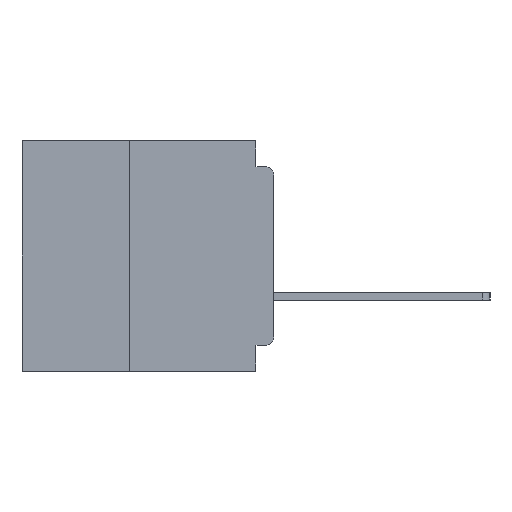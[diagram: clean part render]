
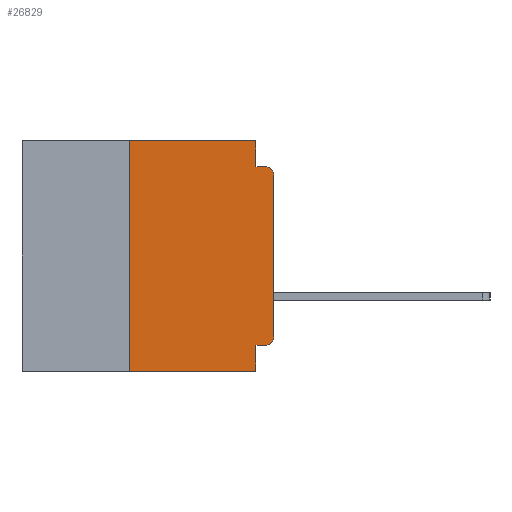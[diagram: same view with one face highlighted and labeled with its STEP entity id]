
A CAD part, left-side view. The second image highlights one B-rep face of the part: STEP entity #26829.
In plain terms, the highlighted planar face has unit normal (-1, 0, 0).
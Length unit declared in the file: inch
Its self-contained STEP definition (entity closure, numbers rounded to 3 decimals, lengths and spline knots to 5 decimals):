
#3 = VERTEX_POINT ( 'NONE', #35363 ) ;
#41 = EDGE_CURVE ( 'NONE', #34626, #41561, #30622, .T. ) ;
#178 = ORIENTED_EDGE ( 'NONE', *, *, #27893, .F. ) ;
#1180 = CARTESIAN_POINT ( 'NONE',  ( 0., 0., -0.06 ) ) ;
#1200 = DIRECTION ( 'NONE',  ( 0., 0., -1. ) ) ;
#1345 = VERTEX_POINT ( 'NONE', #44068 ) ;
#2006 = ORIENTED_EDGE ( 'NONE', *, *, #9228, .F. ) ;
#2143 = CARTESIAN_POINT ( 'NONE',  ( 0., 0.031, 0. ) ) ;
#2938 = EDGE_LOOP ( 'NONE', ( #5595, #6487, #9925, #178, #2006, #3854, #11358, #15460, #45734, #35679 ) ) ;
#3104 = DIRECTION ( 'NONE',  ( 0., 1., 0. ) ) ;
#3542 = VECTOR ( 'NONE', #44884, 39.37008 ) ;
#3665 = DIRECTION ( 'NONE',  ( 1., 0., 0. ) ) ;
#3854 = ORIENTED_EDGE ( 'NONE', *, *, #25334, .F. ) ;
#4952 = VERTEX_POINT ( 'NONE', #33995 ) ;
#5595 = ORIENTED_EDGE ( 'NONE', *, *, #14968, .T. ) ;
#6020 = LINE ( 'NONE', #2143, #12818 ) ;
#6022 = LINE ( 'NONE', #37844, #16567 ) ;
#6487 = ORIENTED_EDGE ( 'NONE', *, *, #41, .T. ) ;
#7938 = VERTEX_POINT ( 'NONE', #29841 ) ;
#8248 = CARTESIAN_POINT ( 'NONE',  ( 0., 0.015, -0.06 ) ) ;
#9228 = EDGE_CURVE ( 'NONE', #7938, #15214, #11077, .T. ) ;
#9925 = ORIENTED_EDGE ( 'NONE', *, *, #34168, .F. ) ;
#10489 = CARTESIAN_POINT ( 'NONE',  ( 0., 0., 0. ) ) ;
#10642 = EDGE_CURVE ( 'NONE', #3, #43529, #35907, .T. ) ;
#11077 = LINE ( 'NONE', #41957, #29340 ) ;
#11358 = ORIENTED_EDGE ( 'NONE', *, *, #14880, .T. ) ;
#12048 = CARTESIAN_POINT ( 'NONE',  ( 0., 0.031, 0. ) ) ;
#12239 = EDGE_CURVE ( 'NONE', #43529, #1345, #24735, .T. ) ;
#12464 = DIRECTION ( 'NONE',  ( -1., 0., 0. ) ) ;
#12818 = VECTOR ( 'NONE', #44821, 39.37008 ) ;
#13395 = CARTESIAN_POINT ( 'NONE',  ( 0., 0., -0.34 ) ) ;
#14012 = VECTOR ( 'NONE', #3104, 39.37008 ) ;
#14355 = LINE ( 'NONE', #20698, #33811 ) ;
#14684 = CARTESIAN_POINT ( 'NONE',  ( 0., 0., -0.355 ) ) ;
#14880 = EDGE_CURVE ( 'NONE', #29068, #1345, #24453, .T. ) ;
#14968 = EDGE_CURVE ( 'NONE', #15480, #34626, #40204, .T. ) ;
#15214 = VERTEX_POINT ( 'NONE', #12048 ) ;
#15460 = ORIENTED_EDGE ( 'NONE', *, *, #12239, .F. ) ;
#15480 = VERTEX_POINT ( 'NONE', #13395 ) ;
#15895 = CARTESIAN_POINT ( 'NONE',  ( 0., 0.015, -0.34 ) ) ;
#16567 = VECTOR ( 'NONE', #41550, 39.37008 ) ;
#17595 = CARTESIAN_POINT ( 'NONE',  ( 0., 0.25, -0.4 ) ) ;
#19838 = DIRECTION ( 'NONE',  ( 0., 0., -1. ) ) ;
#20698 = CARTESIAN_POINT ( 'NONE',  ( 0., 0.25, -0.4 ) ) ;
#20819 = VECTOR ( 'NONE', #33852, 39.37008 ) ;
#22520 = AXIS2_PLACEMENT_3D ( 'NONE', #8248, #12464, #36124 ) ;
#23288 = PLANE ( 'NONE',  #43903 ) ;
#23530 = VECTOR ( 'NONE', #1200, 39.37008 ) ;
#23968 = FACE_OUTER_BOUND ( 'NONE', #2938, .T. ) ;
#24453 = LINE ( 'NONE', #29423, #3542 ) ;
#24594 = DIRECTION ( 'NONE',  ( 0., 0., 1. ) ) ;
#24735 = LINE ( 'NONE', #36448, #23530 ) ;
#25334 = EDGE_CURVE ( 'NONE', #29068, #7938, #14355, .T. ) ;
#26829 = ADVANCED_FACE ( 'NONE', ( #23968 ), #23288, .F. ) ;
#27163 = CARTESIAN_POINT ( 'NONE',  ( 0., 0.437, 0. ) ) ;
#27893 = EDGE_CURVE ( 'NONE', #15214, #4952, #6020, .T. ) ;
#29068 = VERTEX_POINT ( 'NONE', #17595 ) ;
#29340 = VECTOR ( 'NONE', #38078, 39.37008 ) ;
#29423 = CARTESIAN_POINT ( 'NONE',  ( 0., 0.437, -0.4 ) ) ;
#29841 = CARTESIAN_POINT ( 'NONE',  ( 0., 0.25, 0. ) ) ;
#30622 = CIRCLE ( 'NONE', #22520, 0.015 ) ;
#30967 = CARTESIAN_POINT ( 'NONE',  ( 0., 0.015, -0.045 ) ) ;
#31050 = DIRECTION ( 'NONE',  ( 0., 0., -1. ) ) ;
#31498 = CIRCLE ( 'NONE', #33887, 0.015 ) ;
#33560 = CARTESIAN_POINT ( 'NONE',  ( 0., 0.031, -0.355 ) ) ;
#33811 = VECTOR ( 'NONE', #24594, 39.37008 ) ;
#33852 = DIRECTION ( 'NONE',  ( 0., 0., 1. ) ) ;
#33887 = AXIS2_PLACEMENT_3D ( 'NONE', #15895, #43037, #19838 ) ;
#33995 = CARTESIAN_POINT ( 'NONE',  ( 0., 0.031, -0.045 ) ) ;
#34168 = EDGE_CURVE ( 'NONE', #4952, #41561, #6022, .T. ) ;
#34626 = VERTEX_POINT ( 'NONE', #1180 ) ;
#35363 = CARTESIAN_POINT ( 'NONE',  ( 0., 0.015, -0.355 ) ) ;
#35679 = ORIENTED_EDGE ( 'NONE', *, *, #37758, .T. ) ;
#35907 = LINE ( 'NONE', #14684, #14012 ) ;
#36124 = DIRECTION ( 'NONE',  ( 0., 0., -1. ) ) ;
#36448 = CARTESIAN_POINT ( 'NONE',  ( 0., 0.031, -0.4 ) ) ;
#37758 = EDGE_CURVE ( 'NONE', #3, #15480, #31498, .T. ) ;
#37844 = CARTESIAN_POINT ( 'NONE',  ( 0., 0., -0.045 ) ) ;
#38078 = DIRECTION ( 'NONE',  ( 0., -1., 0. ) ) ;
#40204 = LINE ( 'NONE', #10489, #20819 ) ;
#41550 = DIRECTION ( 'NONE',  ( 0., -1., 0. ) ) ;
#41561 = VERTEX_POINT ( 'NONE', #30967 ) ;
#41957 = CARTESIAN_POINT ( 'NONE',  ( 0., 0.437, 0. ) ) ;
#43037 = DIRECTION ( 'NONE',  ( -1., 0., 0. ) ) ;
#43529 = VERTEX_POINT ( 'NONE', #33560 ) ;
#43903 = AXIS2_PLACEMENT_3D ( 'NONE', #27163, #3665, #31050 ) ;
#44068 = CARTESIAN_POINT ( 'NONE',  ( 0., 0.031, -0.4 ) ) ;
#44821 = DIRECTION ( 'NONE',  ( 0., 0., -1. ) ) ;
#44884 = DIRECTION ( 'NONE',  ( 0., -1., 0. ) ) ;
#45734 = ORIENTED_EDGE ( 'NONE', *, *, #10642, .F. ) ;
